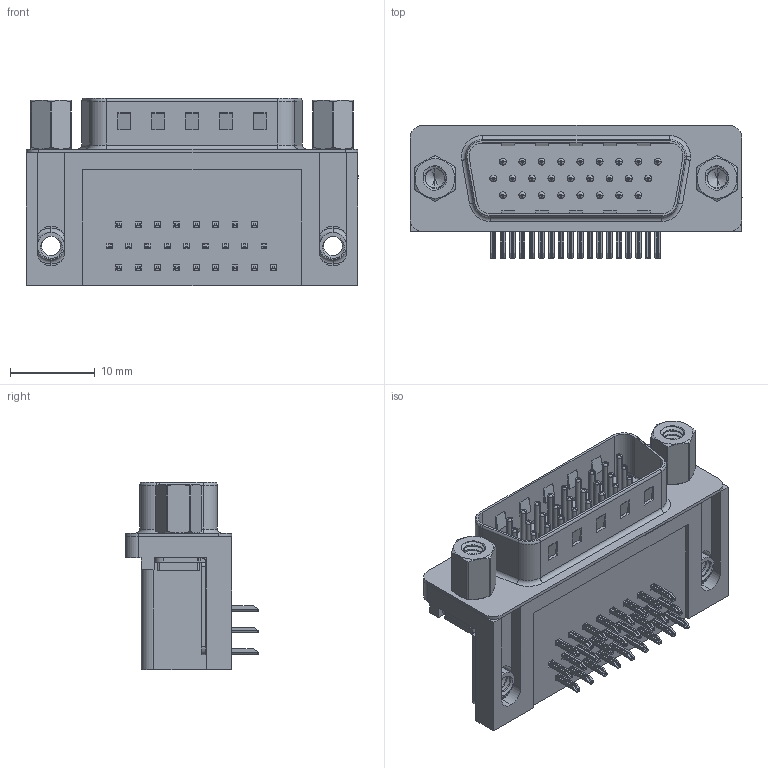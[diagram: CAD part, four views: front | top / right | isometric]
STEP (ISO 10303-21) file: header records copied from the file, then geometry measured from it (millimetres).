
FILE_DESCRIPTION (( 'STEP AP203' ), '1' );
FILE_NAME ('633-026-363-053.STEP', '2018-11-09T00:22:47', ( '' ), ( '' ), 'SwSTEP 2.0', 'SolidWorks 2016', '' );
FILE_SCHEMA (( 'CONFIG_CONTROL_DESIGN' ));
Length unit declared in the file: millimetre
Products named in the file (9): 633 Contact Bottom; 633 Contact Middle; 633 Contact Top; 633 4-40 Threaded Board Mount; 633 4-40 Threaded Rivet; 633 4-40 Hex Standoff; 633-026-363-053; 633 Housing_26 Contact; 633 Shell_26 Contact
Assembly tree (34 placements, depth 2):
  633-026-363-053
    633 Housing_26 Contact
    633 Shell_26 Contact
    633 Contact Bottom  x8
    633 Contact Middle  x9
    633 Contact Top  x9
    633 4-40 Threaded Board Mount  x2
    633 4-40 Threaded Rivet  x2
    633 4-40 Hex Standoff  x2
Bounding box: 39.22 x 15.73 x 22.1 mm (x, y, z)
Volume: 5812 mm3; surface area: 7783.1 mm2
Topology: 34 solids, 34 shells, 2454 faces, 6106 edges, 3781 vertices
Faces by surface type: plane 1443, cylinder 754, torus 199, cone 34, bspline 24
Entity records: 29906 total; most frequent: CARTESIAN_POINT 9682, DIRECTION 3889, ORIENTED_EDGE 3846, EDGE_CURVE 1923, AXIS2_PLACEMENT_3D 1328, VECTOR 1233, LINE 1233, VERTEX_POINT 1231
